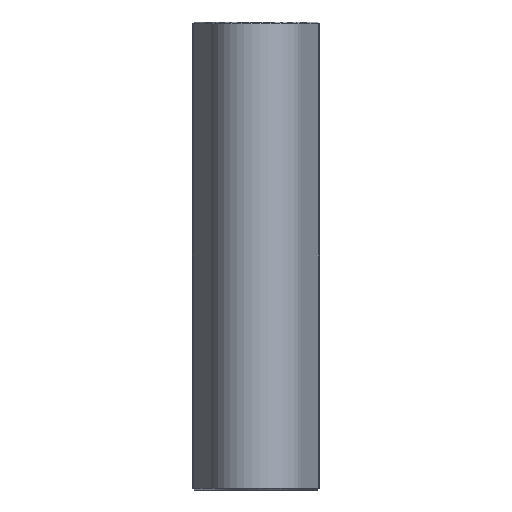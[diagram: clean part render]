
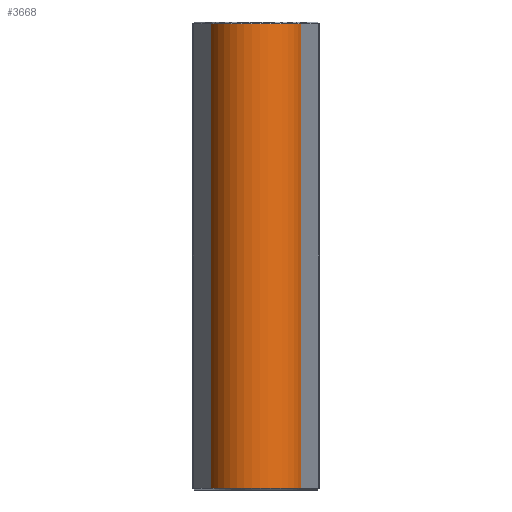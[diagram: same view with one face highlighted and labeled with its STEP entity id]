
A CAD part, front view. The second image highlights one B-rep face of the part: STEP entity #3668.
In plain terms, the highlighted cylindrical face has radius 10 mm (diameter 20 mm), a partial arc.
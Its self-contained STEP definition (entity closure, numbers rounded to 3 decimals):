
#162=CYLINDRICAL_SURFACE('',#4024,10.);
#385=FACE_OUTER_BOUND('',#609,.T.);
#609=EDGE_LOOP('',(#2917,#2918,#2919,#2920));
#741=CIRCLE('',#3810,10.);
#821=CIRCLE('',#3981,10.);
#1092=LINE('',#6081,#1390);
#1093=LINE('',#6083,#1391);
#1390=VECTOR('',#4844,10.);
#1391=VECTOR('',#4847,10.);
#1499=VERTEX_POINT('',#5329);
#1501=VERTEX_POINT('',#5335);
#1691=VERTEX_POINT('',#5915);
#1693=VERTEX_POINT('',#5921);
#1838=EDGE_CURVE('',#1501,#1499,#741,.T.);
#2107=EDGE_CURVE('',#1693,#1691,#821,.T.);
#2172=EDGE_CURVE('',#1691,#1501,#1092,.T.);
#2173=EDGE_CURVE('',#1693,#1499,#1093,.T.);
#2917=ORIENTED_EDGE('',*,*,#1838,.F.);
#2918=ORIENTED_EDGE('',*,*,#2172,.F.);
#2919=ORIENTED_EDGE('',*,*,#2107,.F.);
#2920=ORIENTED_EDGE('',*,*,#2173,.T.);
#3668=ADVANCED_FACE('',(#385),#162,.T.);
#3810=AXIS2_PLACEMENT_3D('',#5337,#4228,#4229);
#3981=AXIS2_PLACEMENT_3D('',#5923,#4729,#4730);
#4024=AXIS2_PLACEMENT_3D('',#6082,#4845,#4846);
#4228=DIRECTION('center_axis',(0.,0.,1.));
#4229=DIRECTION('ref_axis',(1.,0.,0.));
#4729=DIRECTION('center_axis',(0.,0.,-1.));
#4730=DIRECTION('ref_axis',(1.,0.,0.));
#4844=DIRECTION('',(0.,0.,1.));
#4845=DIRECTION('center_axis',(0.,0.,1.));
#4846=DIRECTION('ref_axis',(1.,0.,0.));
#4847=DIRECTION('',(0.,0.,1.));
#5329=CARTESIAN_POINT('',(23.066,-15.914,99.6));
#5335=CARTESIAN_POINT('',(3.934,-15.914,99.6));
#5337=CARTESIAN_POINT('Origin',(13.5,-13.,99.6));
#5915=CARTESIAN_POINT('',(3.934,-15.914,0.4));
#5921=CARTESIAN_POINT('',(23.066,-15.914,0.4));
#5923=CARTESIAN_POINT('Origin',(13.5,-13.,0.4));
#6081=CARTESIAN_POINT('',(3.934,-15.914,0.));
#6082=CARTESIAN_POINT('Origin',(13.5,-13.,0.));
#6083=CARTESIAN_POINT('',(23.066,-15.914,0.));
